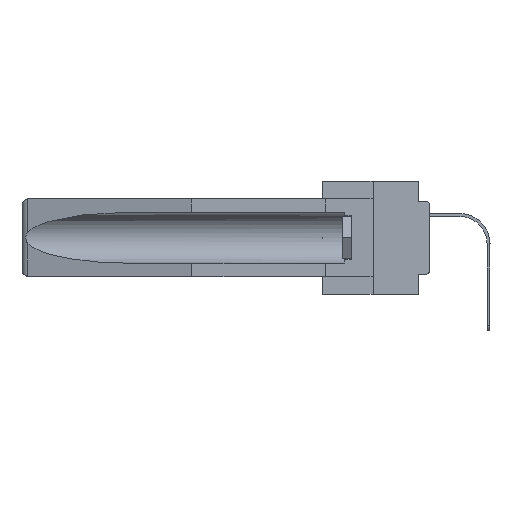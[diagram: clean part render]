
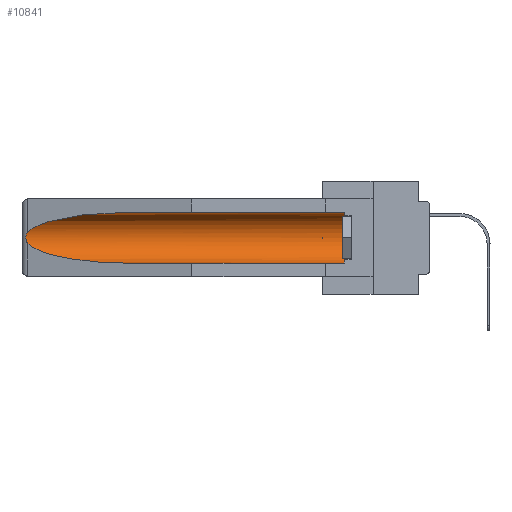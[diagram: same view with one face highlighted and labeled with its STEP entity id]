
A CAD part, left-side view. The second image highlights one B-rep face of the part: STEP entity #10841.
In plain terms, the highlighted cylindrical face has radius 2.857 mm (diameter 5.715 mm), a partial arc.
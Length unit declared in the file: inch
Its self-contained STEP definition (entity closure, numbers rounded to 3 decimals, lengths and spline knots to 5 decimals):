
#120 = AXIS2_PLACEMENT_3D ( 'NONE', #35784, #9084, #32841 ) ;
#566 = CARTESIAN_POINT ( 'NONE',  ( 0.155, 0.126, -0.284 ) ) ;
#2477 = VERTEX_POINT ( 'NONE', #33512 ) ;
#2657 = CARTESIAN_POINT ( 'NONE',  ( 0.155, 1.07973, -0.284 ) ) ;
#3657 = EDGE_LOOP ( 'NONE', ( #33793, #25322, #16490, #24725, #28621, #36587 ) ) ;
#3823 = CARTESIAN_POINT ( 'NONE',  ( 0.26537, 1.52718, -0.14972 ) ) ;
#4882 = DIRECTION ( 'NONE',  ( 0., 1., 0. ) ) ;
#5083 = CARTESIAN_POINT ( 'NONE',  ( 0.26537, 1.52718, -0.19328 ) ) ;
#5257 = CARTESIAN_POINT ( 'NONE',  ( 0.26537, 1.52718, -0.19328 ) ) ;
#5570 = CARTESIAN_POINT ( 'NONE',  ( 0.26537, 1.52718, -0.19328 ) ) ;
#5881 = VERTEX_POINT ( 'NONE', #566 ) ;
#7513 = B_SPLINE_CURVE_WITH_KNOTS ( 'NONE', 3,
 ( #23424, #29649, #35687, #35489, #35299, #28875, #14265, #23813, #35113, #5257 ),
 .UNSPECIFIED., .F., .F.,
 ( 4, 2, 2, 2, 4 ),
 ( 0., 0.00029, 0.00058, 0.00087, 0.00117 ),
 .UNSPECIFIED. ) ;
#7642 = DIRECTION ( 'NONE',  ( 0., 0., 1. ) ) ;
#8028 = CYLINDRICAL_SURFACE ( 'NONE', #38033, 0.1125 ) ;
#8889 = EDGE_CURVE ( 'NONE', #5881, #16897, #18834, .T. ) ;
#9084 = DIRECTION ( 'NONE',  ( 0., -1., 0. ) ) ;
#9534 = VERTEX_POINT ( 'NONE', #5083 ) ;
#10841 = ADVANCED_FACE ( 'NONE', ( #22278 ), #8028, .F. ) ;
#11851 = CARTESIAN_POINT ( 'NONE',  ( 0.25451, 1.48313, -0.24835 ) ) ;
#12246 = CARTESIAN_POINT ( 'NONE',  ( 0.155, -0.30754, -0.284 ) ) ;
#14265 = CARTESIAN_POINT ( 'NONE',  ( 0.2673, 1.53269, -0.17917 ) ) ;
#15180 = LINE ( 'NONE', #12246, #17144 ) ;
#15595 = DIRECTION ( 'NONE',  ( 0., 1., 0. ) ) ;
#16490 = ORIENTED_EDGE ( 'NONE', *, *, #25095, .T. ) ;
#16897 = VERTEX_POINT ( 'NONE', #37412 ) ;
#17144 = VECTOR ( 'NONE', #22356, 39.37008 ) ;
#17159 = EDGE_CURVE ( 'NONE', #17176, #20231, #36295, .T. ) ;
#17176 = VERTEX_POINT ( 'NONE', #36216 ) ;
#17523 = VECTOR ( 'NONE', #15595, 39.37008 ) ;
#18834 = CIRCLE ( 'NONE', #120, 0.1125 ) ;
#20231 = VERTEX_POINT ( 'NONE', #21498 ) ;
#21498 = CARTESIAN_POINT ( 'NONE',  ( 0.26537, 1.52718, -0.14972 ) ) ;
#22002 = EDGE_CURVE ( 'NONE', #16897, #17176, #24163, .T. ) ;
#22278 = FACE_OUTER_BOUND ( 'NONE', #3657, .T. ) ;
#22356 = DIRECTION ( 'NONE',  ( 0., 1., 0. ) ) ;
#23424 = CARTESIAN_POINT ( 'NONE',  ( 0.26537, 1.52718, -0.14972 ) ) ;
#23813 = CARTESIAN_POINT ( 'NONE',  ( 0.26655, 1.53094, -0.18657 ) ) ;
#24163 = LINE ( 'NONE', #29315, #17523 ) ;
#24725 = ORIENTED_EDGE ( 'NONE', *, *, #29458, .F. ) ;
#25095 = EDGE_CURVE ( 'NONE', #9534, #2477, #38578, .T. ) ;
#25322 = ORIENTED_EDGE ( 'NONE', *, *, #28762, .T. ) ;
#28621 = ORIENTED_EDGE ( 'NONE', *, *, #8889, .T. ) ;
#28762 = EDGE_CURVE ( 'NONE', #20231, #9534, #7513, .T. ) ;
#28875 = CARTESIAN_POINT ( 'NONE',  ( 0.2675, 1.53308, -0.17534 ) ) ;
#29315 = CARTESIAN_POINT ( 'NONE',  ( 0.155, -0.30754, -0.059 ) ) ;
#29458 = EDGE_CURVE ( 'NONE', #5881, #2477, #15180, .T. ) ;
#29649 = CARTESIAN_POINT ( 'NONE',  ( 0.26597, 1.52961, -0.15275 ) ) ;
#29979 = CARTESIAN_POINT ( 'NONE',  ( 0.25451, 1.48313, -0.09465 ) ) ;
#32841 = DIRECTION ( 'NONE',  ( 0., 0., 1. ) ) ;
#33089 = CARTESIAN_POINT ( 'NONE',  ( 0.21114, 1.30732, -0.059 ) ) ;
#33456 = CARTESIAN_POINT ( 'NONE',  ( 0.155, 1.07973, -0.059 ) ) ;
#33512 = CARTESIAN_POINT ( 'NONE',  ( 0.155, 1.07973, -0.284 ) ) ;
#33793 = ORIENTED_EDGE ( 'NONE', *, *, #17159, .T. ) ;
#34354 = CARTESIAN_POINT ( 'NONE',  ( 0.155, -0.30754, -0.1715 ) ) ;
#35113 = CARTESIAN_POINT ( 'NONE',  ( 0.26597, 1.5296, -0.19026 ) ) ;
#35299 = CARTESIAN_POINT ( 'NONE',  ( 0.2675, 1.53308, -0.16763 ) ) ;
#35489 = CARTESIAN_POINT ( 'NONE',  ( 0.2673, 1.5327, -0.16383 ) ) ;
#35687 = CARTESIAN_POINT ( 'NONE',  ( 0.26654, 1.53092, -0.15636 ) ) ;
#35784 = CARTESIAN_POINT ( 'NONE',  ( 0.155, 0.126, -0.1715 ) ) ;
#36216 = CARTESIAN_POINT ( 'NONE',  ( 0.155, 1.07973, -0.059 ) ) ;
#36295 =( BOUNDED_CURVE ( )  B_SPLINE_CURVE ( 3, ( #33456, #33089, #29979, #3823 ),
 .UNSPECIFIED., .F., .F. ) 
 B_SPLINE_CURVE_WITH_KNOTS ( ( 4, 4 ),
 ( 4.71239, 6.08839 ),
 .UNSPECIFIED. ) 
 CURVE ( )  GEOMETRIC_REPRESENTATION_ITEM ( )  RATIONAL_B_SPLINE_CURVE ( ( 1., 0.848, 0.848, 1. ) ) 
 REPRESENTATION_ITEM ( '' )  );
#36587 = ORIENTED_EDGE ( 'NONE', *, *, #22002, .T. ) ;
#37412 = CARTESIAN_POINT ( 'NONE',  ( 0.155, 0.126, -0.059 ) ) ;
#38033 = AXIS2_PLACEMENT_3D ( 'NONE', #34354, #4882, #7642 ) ;
#38547 = CARTESIAN_POINT ( 'NONE',  ( 0.21114, 1.30732, -0.284 ) ) ;
#38578 =( BOUNDED_CURVE ( )  B_SPLINE_CURVE ( 3, ( #5570, #11851, #38547, #2657 ),
 .UNSPECIFIED., .F., .F. ) 
 B_SPLINE_CURVE_WITH_KNOTS ( ( 4, 4 ),
 ( 0.1948, 1.5708 ),
 .UNSPECIFIED. ) 
 CURVE ( )  GEOMETRIC_REPRESENTATION_ITEM ( )  RATIONAL_B_SPLINE_CURVE ( ( 1., 0.848, 0.848, 1. ) ) 
 REPRESENTATION_ITEM ( '' )  );
